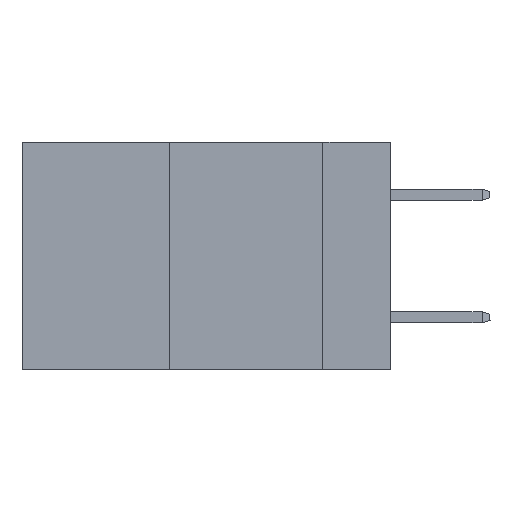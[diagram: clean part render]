
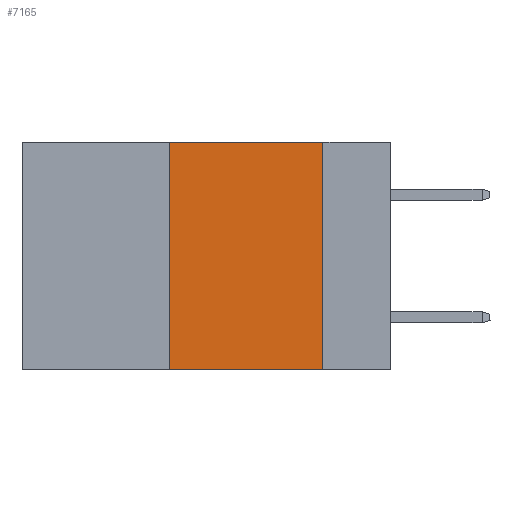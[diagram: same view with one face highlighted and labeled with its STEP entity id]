
A CAD part, left-side view. The second image highlights one B-rep face of the part: STEP entity #7165.
In plain terms, the highlighted planar face has unit normal (-1, 0, 0).
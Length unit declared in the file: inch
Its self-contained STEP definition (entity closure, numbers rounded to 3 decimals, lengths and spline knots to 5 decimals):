
#385 = VERTEX_POINT ( 'NONE', #3837 ) ;
#431 = ORIENTED_EDGE ( 'NONE', *, *, #15463, .F. ) ;
#514 = CARTESIAN_POINT ( 'NONE',  ( 0., 0.36, -0.37 ) ) ;
#2340 = EDGE_CURVE ( 'NONE', #20709, #385, #26186, .T. ) ;
#2363 = EDGE_LOOP ( 'NONE', ( #431, #9698, #7033, #23390 ) ) ;
#2471 = LINE ( 'NONE', #24428, #18681 ) ;
#3541 = DIRECTION ( 'NONE',  ( 0., -1., 0. ) ) ;
#3837 = CARTESIAN_POINT ( 'NONE',  ( 0., 0.36, 0. ) ) ;
#4153 = VECTOR ( 'NONE', #3541, 39.37008 ) ;
#6353 = VERTEX_POINT ( 'NONE', #25200 ) ;
#6992 = VECTOR ( 'NONE', #16217, 39.37008 ) ;
#7033 = ORIENTED_EDGE ( 'NONE', *, *, #2340, .F. ) ;
#7165 = ADVANCED_FACE ( 'NONE', ( #18533 ), #11377, .F. ) ;
#9698 = ORIENTED_EDGE ( 'NONE', *, *, #10768, .F. ) ;
#10768 = EDGE_CURVE ( 'NONE', #385, #25791, #2471, .T. ) ;
#10836 = EDGE_CURVE ( 'NONE', #20709, #6353, #19025, .T. ) ;
#11377 = PLANE ( 'NONE',  #23310 ) ;
#11522 = CARTESIAN_POINT ( 'NONE',  ( 0., 0.11, 0. ) ) ;
#14606 = CARTESIAN_POINT ( 'NONE',  ( 0., 0.36, 0. ) ) ;
#15463 = EDGE_CURVE ( 'NONE', #25791, #6353, #15581, .T. ) ;
#15581 = LINE ( 'NONE', #11522, #6992 ) ;
#15631 = DIRECTION ( 'NONE',  ( 0., 0., -1. ) ) ;
#16217 = DIRECTION ( 'NONE',  ( 0., 0., -1. ) ) ;
#16818 = DIRECTION ( 'NONE',  ( 0., 0., 1. ) ) ;
#17931 = CARTESIAN_POINT ( 'NONE',  ( 0., 0.6, 0. ) ) ;
#18533 = FACE_OUTER_BOUND ( 'NONE', #2363, .T. ) ;
#18681 = VECTOR ( 'NONE', #24616, 39.37008 ) ;
#19025 = LINE ( 'NONE', #26467, #4153 ) ;
#20563 = VECTOR ( 'NONE', #16818, 39.37008 ) ;
#20709 = VERTEX_POINT ( 'NONE', #514 ) ;
#22258 = DIRECTION ( 'NONE',  ( 1., 0., 0. ) ) ;
#23310 = AXIS2_PLACEMENT_3D ( 'NONE', #17931, #22258, #15631 ) ;
#23390 = ORIENTED_EDGE ( 'NONE', *, *, #10836, .T. ) ;
#24428 = CARTESIAN_POINT ( 'NONE',  ( 0., 0.6, 0. ) ) ;
#24616 = DIRECTION ( 'NONE',  ( 0., -1., 0. ) ) ;
#24919 = CARTESIAN_POINT ( 'NONE',  ( 0., 0.11, 0. ) ) ;
#25200 = CARTESIAN_POINT ( 'NONE',  ( 0., 0.11, -0.37 ) ) ;
#25791 = VERTEX_POINT ( 'NONE', #24919 ) ;
#26186 = LINE ( 'NONE', #14606, #20563 ) ;
#26467 = CARTESIAN_POINT ( 'NONE',  ( 0., 0.6, -0.37 ) ) ;
